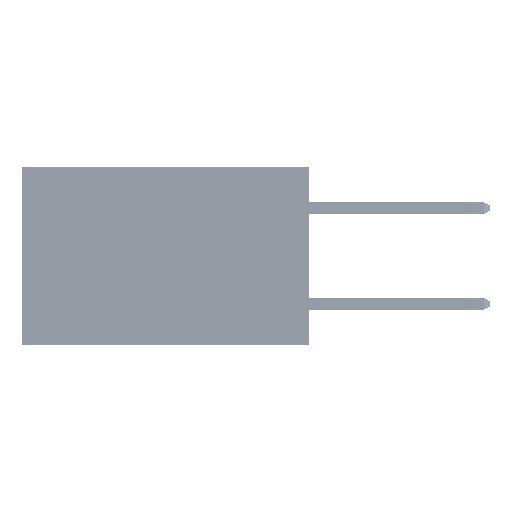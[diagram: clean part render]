
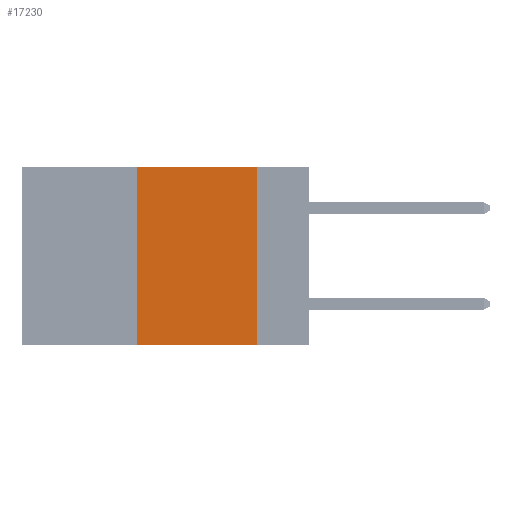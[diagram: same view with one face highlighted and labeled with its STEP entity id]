
A CAD part, left-side view. The second image highlights one B-rep face of the part: STEP entity #17230.
In plain terms, the highlighted planar face has unit normal (-1, 0, 0).
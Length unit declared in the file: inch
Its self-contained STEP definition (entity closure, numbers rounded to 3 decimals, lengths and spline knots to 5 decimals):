
#2273 = EDGE_CURVE ( 'NONE', #6999, #6388, #17751, .T. ) ;
#3626 = EDGE_CURVE ( 'NONE', #43776, #6388, #17989, .T. ) ;
#4119 = ORIENTED_EDGE ( 'NONE', *, *, #23010, .F. ) ;
#5291 = DIRECTION ( 'NONE',  ( 0., -1., 0. ) ) ;
#5884 = CARTESIAN_POINT ( 'NONE',  ( 0., 0.11, 0. ) ) ;
#6076 = DIRECTION ( 'NONE',  ( 0., 0., -1. ) ) ;
#6388 = VERTEX_POINT ( 'NONE', #30632 ) ;
#6410 = LINE ( 'NONE', #19657, #31432 ) ;
#6859 = VECTOR ( 'NONE', #8780, 39.37008 ) ;
#6999 = VERTEX_POINT ( 'NONE', #46549 ) ;
#7765 = AXIS2_PLACEMENT_3D ( 'NONE', #13283, #17413, #46089 ) ;
#8780 = DIRECTION ( 'NONE',  ( 0., -1., 0. ) ) ;
#9321 = PLANE ( 'NONE',  #7765 ) ;
#12075 = EDGE_CURVE ( 'NONE', #6999, #26644, #6410, .T. ) ;
#12741 = CARTESIAN_POINT ( 'NONE',  ( 0., 0.6, 0. ) ) ;
#13283 = CARTESIAN_POINT ( 'NONE',  ( 0., 0.6, 0. ) ) ;
#16510 = ORIENTED_EDGE ( 'NONE', *, *, #2273, .T. ) ;
#17230 = ADVANCED_FACE ( 'NONE', ( #42557 ), #9321, .F. ) ;
#17413 = DIRECTION ( 'NONE',  ( 1., 0., 0. ) ) ;
#17751 = LINE ( 'NONE', #33488, #38247 ) ;
#17989 = LINE ( 'NONE', #5884, #32070 ) ;
#19355 = CARTESIAN_POINT ( 'NONE',  ( 0., 0.36, 0. ) ) ;
#19657 = CARTESIAN_POINT ( 'NONE',  ( 0., 0.36, 0. ) ) ;
#23010 = EDGE_CURVE ( 'NONE', #26644, #43776, #37024, .T. ) ;
#26059 = CARTESIAN_POINT ( 'NONE',  ( 0., 0.11, 0. ) ) ;
#26644 = VERTEX_POINT ( 'NONE', #19355 ) ;
#30632 = CARTESIAN_POINT ( 'NONE',  ( 0., 0.11, -0.37 ) ) ;
#31432 = VECTOR ( 'NONE', #47793, 39.37008 ) ;
#32070 = VECTOR ( 'NONE', #6076, 39.37008 ) ;
#33488 = CARTESIAN_POINT ( 'NONE',  ( 0., 0.6, -0.37 ) ) ;
#37024 = LINE ( 'NONE', #12741, #6859 ) ;
#38247 = VECTOR ( 'NONE', #5291, 39.37008 ) ;
#42549 = EDGE_LOOP ( 'NONE', ( #51194, #4119, #50009, #16510 ) ) ;
#42557 = FACE_OUTER_BOUND ( 'NONE', #42549, .T. ) ;
#43776 = VERTEX_POINT ( 'NONE', #26059 ) ;
#46089 = DIRECTION ( 'NONE',  ( 0., 0., -1. ) ) ;
#46549 = CARTESIAN_POINT ( 'NONE',  ( 0., 0.36, -0.37 ) ) ;
#47793 = DIRECTION ( 'NONE',  ( 0., 0., 1. ) ) ;
#50009 = ORIENTED_EDGE ( 'NONE', *, *, #12075, .F. ) ;
#51194 = ORIENTED_EDGE ( 'NONE', *, *, #3626, .F. ) ;
